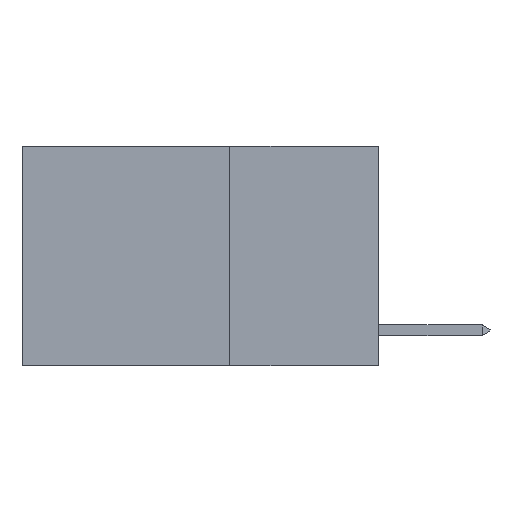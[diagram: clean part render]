
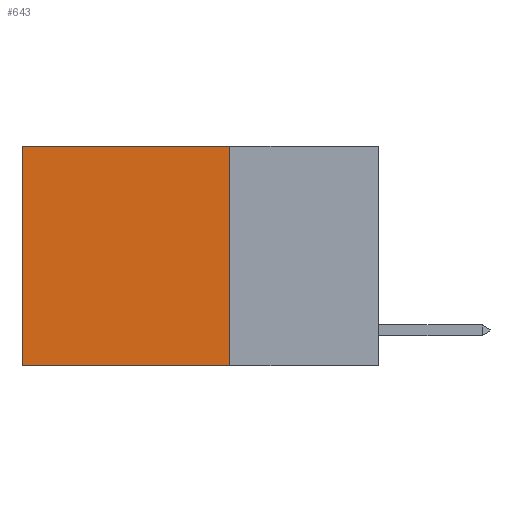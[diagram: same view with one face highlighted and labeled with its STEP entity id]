
A CAD part, left-side view. The second image highlights one B-rep face of the part: STEP entity #643.
In plain terms, the highlighted planar face has unit normal (-1, 0, 0).
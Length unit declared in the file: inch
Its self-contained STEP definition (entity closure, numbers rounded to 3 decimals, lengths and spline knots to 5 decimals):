
#323 = VERTEX_POINT ( 'NONE', #5523 ) ;
#416 = DIRECTION ( 'NONE',  ( 0., 1., 0. ) ) ;
#643 = ADVANCED_FACE ( 'NONE', ( #1324 ), #7808, .F. ) ;
#1324 = FACE_OUTER_BOUND ( 'NONE', #15526, .T. ) ;
#1698 = CARTESIAN_POINT ( 'NONE',  ( 0.2625, 0.25, 0. ) ) ;
#1946 = DIRECTION ( 'NONE',  ( 0., 0., -1. ) ) ;
#2158 = CARTESIAN_POINT ( 'NONE',  ( 0.2625, 0.6, -0.37 ) ) ;
#2251 = ORIENTED_EDGE ( 'NONE', *, *, #12218, .F. ) ;
#2267 = DIRECTION ( 'NONE',  ( 0., 0., -1. ) ) ;
#3400 = LINE ( 'NONE', #10956, #10185 ) ;
#3491 = EDGE_CURVE ( 'NONE', #323, #15900, #8505, .T. ) ;
#4210 = DIRECTION ( 'NONE',  ( 0., 1., 0. ) ) ;
#5095 = VERTEX_POINT ( 'NONE', #13806 ) ;
#5523 = CARTESIAN_POINT ( 'NONE',  ( 0.2625, 0.6, 0. ) ) ;
#6686 = DIRECTION ( 'NONE',  ( 1., 0., 0. ) ) ;
#7328 = LINE ( 'NONE', #15878, #9493 ) ;
#7808 = PLANE ( 'NONE',  #14687 ) ;
#8002 = CARTESIAN_POINT ( 'NONE',  ( 0.2625, 0.25, 0. ) ) ;
#8040 = VERTEX_POINT ( 'NONE', #14298 ) ;
#8089 = VECTOR ( 'NONE', #4210, 39.37008 ) ;
#8116 = VECTOR ( 'NONE', #8381, 39.37008 ) ;
#8130 = ORIENTED_EDGE ( 'NONE', *, *, #3491, .T. ) ;
#8381 = DIRECTION ( 'NONE',  ( 0., 0., -1. ) ) ;
#8505 = LINE ( 'NONE', #15969, #8116 ) ;
#9493 = VECTOR ( 'NONE', #416, 39.37008 ) ;
#9860 = EDGE_CURVE ( 'NONE', #8040, #5095, #3400, .T. ) ;
#10185 = VECTOR ( 'NONE', #1946, 39.37008 ) ;
#10956 = CARTESIAN_POINT ( 'NONE',  ( 0.2625, 0.25, 0. ) ) ;
#11343 = ORIENTED_EDGE ( 'NONE', *, *, #9860, .F. ) ;
#12218 = EDGE_CURVE ( 'NONE', #5095, #15900, #7328, .T. ) ;
#13806 = CARTESIAN_POINT ( 'NONE',  ( 0.2625, 0.25, -0.37 ) ) ;
#14128 = ORIENTED_EDGE ( 'NONE', *, *, #14843, .T. ) ;
#14298 = CARTESIAN_POINT ( 'NONE',  ( 0.2625, 0.25, 0. ) ) ;
#14416 = LINE ( 'NONE', #8002, #8089 ) ;
#14687 = AXIS2_PLACEMENT_3D ( 'NONE', #1698, #6686, #2267 ) ;
#14843 = EDGE_CURVE ( 'NONE', #8040, #323, #14416, .T. ) ;
#15526 = EDGE_LOOP ( 'NONE', ( #8130, #2251, #11343, #14128 ) ) ;
#15878 = CARTESIAN_POINT ( 'NONE',  ( 0.2625, 0.25, -0.37 ) ) ;
#15900 = VERTEX_POINT ( 'NONE', #2158 ) ;
#15969 = CARTESIAN_POINT ( 'NONE',  ( 0.2625, 0.6, 0. ) ) ;
